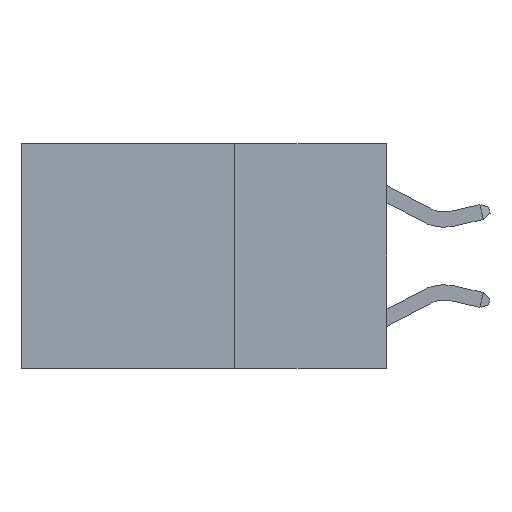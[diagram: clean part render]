
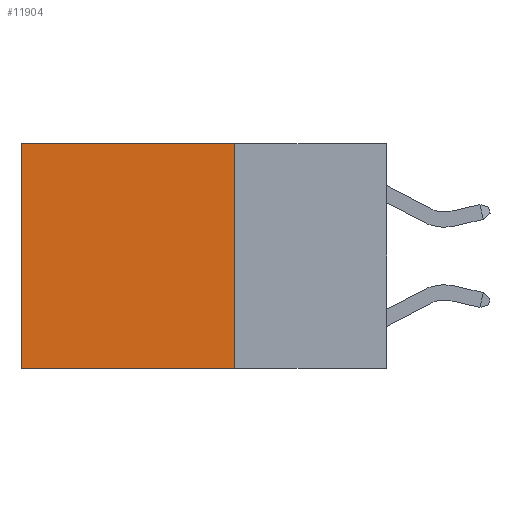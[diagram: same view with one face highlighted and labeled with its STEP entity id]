
A CAD part, left-side view. The second image highlights one B-rep face of the part: STEP entity #11904.
In plain terms, the highlighted planar face has unit normal (-1, 0, 0).
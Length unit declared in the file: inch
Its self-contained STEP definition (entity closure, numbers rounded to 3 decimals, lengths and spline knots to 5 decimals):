
#492 = PLANE ( 'NONE',  #2877 ) ;
#659 = CARTESIAN_POINT ( 'NONE',  ( 0.2625, 0.25, 0. ) ) ;
#940 = EDGE_LOOP ( 'NONE', ( #15078, #17472, #13046, #12201 ) ) ;
#1750 = VECTOR ( 'NONE', #15769, 39.37008 ) ;
#1944 = CARTESIAN_POINT ( 'NONE',  ( 0.2625, 0.25, 0. ) ) ;
#2877 = AXIS2_PLACEMENT_3D ( 'NONE', #13732, #13794, #4994 ) ;
#4570 = VERTEX_POINT ( 'NONE', #6324 ) ;
#4994 = DIRECTION ( 'NONE',  ( 0., 0., -1. ) ) ;
#5543 = CARTESIAN_POINT ( 'NONE',  ( 0.2625, 0.25, -0.37 ) ) ;
#5798 = DIRECTION ( 'NONE',  ( 0., 0., -1. ) ) ;
#6014 = CARTESIAN_POINT ( 'NONE',  ( 0.2625, 0.6, 0. ) ) ;
#6082 = LINE ( 'NONE', #7283, #17254 ) ;
#6324 = CARTESIAN_POINT ( 'NONE',  ( 0.2625, 0.25, -0.37 ) ) ;
#6947 = EDGE_CURVE ( 'NONE', #14367, #14841, #6082, .T. ) ;
#7283 = CARTESIAN_POINT ( 'NONE',  ( 0.2625, 0.6, 0. ) ) ;
#7603 = VERTEX_POINT ( 'NONE', #9233 ) ;
#7681 = EDGE_CURVE ( 'NONE', #7603, #14367, #17221, .T. ) ;
#8519 = CARTESIAN_POINT ( 'NONE',  ( 0.2625, 0.6, -0.37 ) ) ;
#9135 = EDGE_CURVE ( 'NONE', #7603, #4570, #9461, .T. ) ;
#9233 = CARTESIAN_POINT ( 'NONE',  ( 0.2625, 0.25, 0. ) ) ;
#9419 = DIRECTION ( 'NONE',  ( 0., 1., 0. ) ) ;
#9461 = LINE ( 'NONE', #659, #12889 ) ;
#10931 = EDGE_CURVE ( 'NONE', #4570, #14841, #13076, .T. ) ;
#11904 = ADVANCED_FACE ( 'NONE', ( #16857 ), #492, .F. ) ;
#12201 = ORIENTED_EDGE ( 'NONE', *, *, #7681, .T. ) ;
#12499 = DIRECTION ( 'NONE',  ( 0., 0., -1. ) ) ;
#12889 = VECTOR ( 'NONE', #12499, 39.37008 ) ;
#13046 = ORIENTED_EDGE ( 'NONE', *, *, #9135, .F. ) ;
#13076 = LINE ( 'NONE', #5543, #1750 ) ;
#13395 = VECTOR ( 'NONE', #9419, 39.37008 ) ;
#13732 = CARTESIAN_POINT ( 'NONE',  ( 0.2625, 0.25, 0. ) ) ;
#13794 = DIRECTION ( 'NONE',  ( 1., 0., 0. ) ) ;
#14367 = VERTEX_POINT ( 'NONE', #6014 ) ;
#14841 = VERTEX_POINT ( 'NONE', #8519 ) ;
#15078 = ORIENTED_EDGE ( 'NONE', *, *, #6947, .T. ) ;
#15769 = DIRECTION ( 'NONE',  ( 0., 1., 0. ) ) ;
#16857 = FACE_OUTER_BOUND ( 'NONE', #940, .T. ) ;
#17221 = LINE ( 'NONE', #1944, #13395 ) ;
#17254 = VECTOR ( 'NONE', #5798, 39.37008 ) ;
#17472 = ORIENTED_EDGE ( 'NONE', *, *, #10931, .F. ) ;
